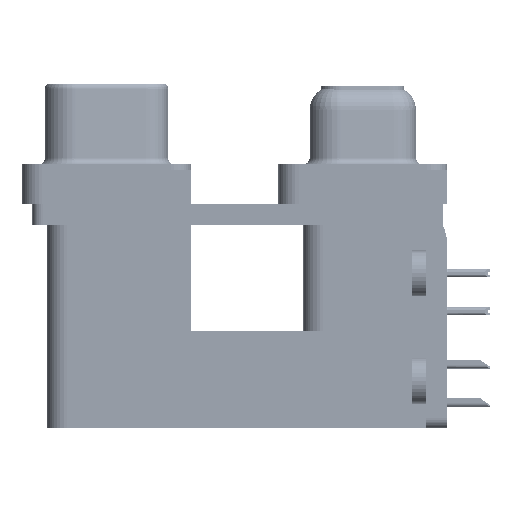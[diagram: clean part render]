
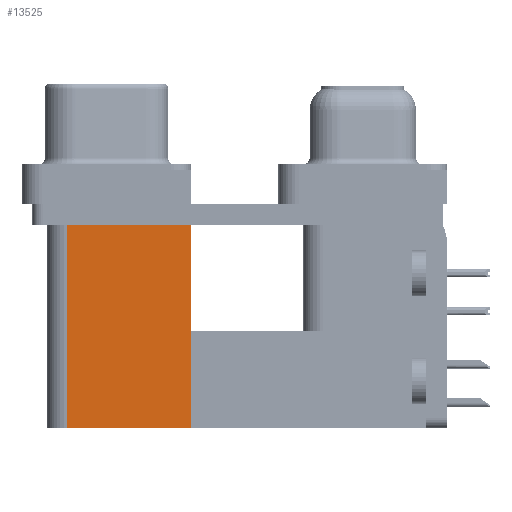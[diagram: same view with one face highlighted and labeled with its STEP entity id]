
A CAD part, left-side view. The second image highlights one B-rep face of the part: STEP entity #13525.
In plain terms, the highlighted planar face has unit normal (-1, 0, 0).
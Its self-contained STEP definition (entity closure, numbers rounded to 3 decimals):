
#2996 = LINE ( 'NONE', #39915, #52384 ) ;
#6371 = ORIENTED_EDGE ( 'NONE', *, *, #11774, .F. ) ;
#6678 = EDGE_CURVE ( 'NONE', #9461, #50000, #11020, .T. ) ;
#6698 = VECTOR ( 'NONE', #25386, 1000. ) ;
#8077 = CARTESIAN_POINT ( 'NONE',  ( 3.79, 12.775, -19.2 ) ) ;
#9014 = DIRECTION ( 'NONE',  ( 0., 1., 0. ) ) ;
#9461 = VERTEX_POINT ( 'NONE', #12180 ) ;
#9560 = DIRECTION ( 'NONE',  ( 0., 1., 0. ) ) ;
#10389 = EDGE_CURVE ( 'NONE', #45718, #9461, #62696, .T. ) ;
#11020 = LINE ( 'NONE', #65649, #22259 ) ;
#11774 = EDGE_CURVE ( 'NONE', #45718, #38366, #2996, .T. ) ;
#12180 = CARTESIAN_POINT ( 'NONE',  ( 3.79, 12.775, -2.5 ) ) ;
#13525 = ADVANCED_FACE ( 'NONE', ( #41852 ), #63490, .F. ) ;
#17023 = DIRECTION ( 'NONE',  ( 0., 1., 0. ) ) ;
#17736 = ORIENTED_EDGE ( 'NONE', *, *, #51913, .F. ) ;
#19018 = LINE ( 'NONE', #23996, #6698 ) ;
#22259 = VECTOR ( 'NONE', #17023, 1000. ) ;
#23956 = CARTESIAN_POINT ( 'NONE',  ( 3.79, 21.975, -2.5 ) ) ;
#23996 = CARTESIAN_POINT ( 'NONE',  ( 3.79, 21.975, -19.2 ) ) ;
#25386 = DIRECTION ( 'NONE',  ( 0., 0., 1. ) ) ;
#33068 = CARTESIAN_POINT ( 'NONE',  ( 3.79, 12.775, -19.2 ) ) ;
#36524 = CARTESIAN_POINT ( 'NONE',  ( 3.79, 12.775, -19.2 ) ) ;
#38366 = VERTEX_POINT ( 'NONE', #58783 ) ;
#39541 = ORIENTED_EDGE ( 'NONE', *, *, #10389, .T. ) ;
#39915 = CARTESIAN_POINT ( 'NONE',  ( 3.79, 12.775, -19.2 ) ) ;
#41852 = FACE_OUTER_BOUND ( 'NONE', #57342, .T. ) ;
#45718 = VERTEX_POINT ( 'NONE', #33068 ) ;
#46016 = ORIENTED_EDGE ( 'NONE', *, *, #6678, .T. ) ;
#50000 = VERTEX_POINT ( 'NONE', #23956 ) ;
#51913 = EDGE_CURVE ( 'NONE', #38366, #50000, #19018, .T. ) ;
#52384 = VECTOR ( 'NONE', #9014, 1000. ) ;
#57342 = EDGE_LOOP ( 'NONE', ( #46016, #17736, #6371, #39541 ) ) ;
#58173 = DIRECTION ( 'NONE',  ( 1., 0., 0. ) ) ;
#58783 = CARTESIAN_POINT ( 'NONE',  ( 3.79, 21.975, -19.2 ) ) ;
#59235 = VECTOR ( 'NONE', #67325, 1000. ) ;
#59802 = AXIS2_PLACEMENT_3D ( 'NONE', #36524, #58173, #9560 ) ;
#62696 = LINE ( 'NONE', #8077, #59235 ) ;
#63490 = PLANE ( 'NONE',  #59802 ) ;
#65649 = CARTESIAN_POINT ( 'NONE',  ( 3.79, 12.775, -2.5 ) ) ;
#67325 = DIRECTION ( 'NONE',  ( 0., 0., 1. ) ) ;
